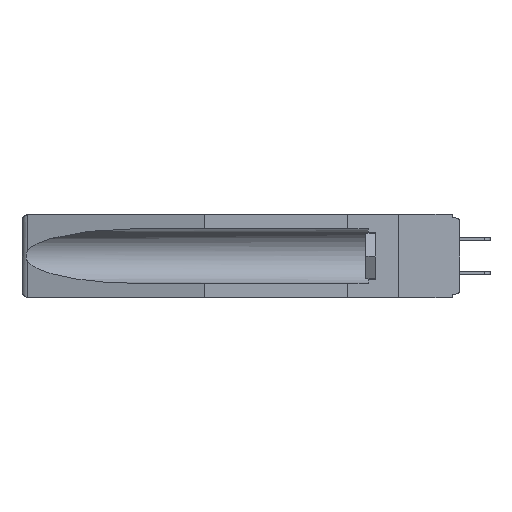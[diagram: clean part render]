
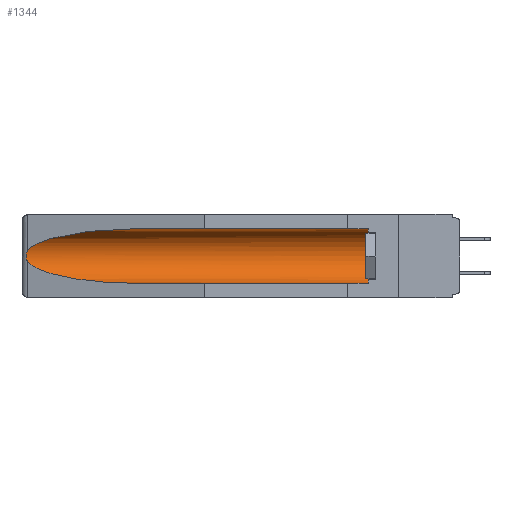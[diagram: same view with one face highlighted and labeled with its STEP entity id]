
A CAD part, left-side view. The second image highlights one B-rep face of the part: STEP entity #1344.
In plain terms, the highlighted cylindrical face has radius 2.857 mm (diameter 5.715 mm), a partial arc.
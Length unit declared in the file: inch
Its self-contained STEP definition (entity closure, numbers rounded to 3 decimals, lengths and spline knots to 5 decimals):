
#11 = LINE ( 'NONE', #16785, #6867 ) ;
#133 = CARTESIAN_POINT ( 'NONE',  ( 0.2673, 1.5327, -0.16383 ) ) ;
#203 = CARTESIAN_POINT ( 'NONE',  ( 0.2673, 1.53269, -0.17917 ) ) ;
#347 = AXIS2_PLACEMENT_3D ( 'NONE', #17643, #7484, #14903 ) ;
#1344 = ADVANCED_FACE ( 'NONE', ( #14683 ), #8242, .F. ) ;
#1616 = CARTESIAN_POINT ( 'NONE',  ( 0.2675, 1.53308, -0.17534 ) ) ;
#1624 = CARTESIAN_POINT ( 'NONE',  ( 0.26537, 1.52718, -0.19328 ) ) ;
#1692 = EDGE_CURVE ( 'NONE', #14448, #6231, #11, .T. ) ;
#2121 = CARTESIAN_POINT ( 'NONE',  ( 0.26537, 1.52718, -0.14972 ) ) ;
#2206 = CARTESIAN_POINT ( 'NONE',  ( 0.25451, 1.48313, -0.09465 ) ) ;
#2249 = DIRECTION ( 'NONE',  ( 0., 1., 0. ) ) ;
#2515 = VERTEX_POINT ( 'NONE', #17437 ) ;
#2989 = LINE ( 'NONE', #17685, #14183 ) ;
#2992 = VERTEX_POINT ( 'NONE', #1624 ) ;
#3052 = CARTESIAN_POINT ( 'NONE',  ( 0.21114, 1.30732, -0.284 ) ) ;
#4793 = CARTESIAN_POINT ( 'NONE',  ( 0.26654, 1.53092, -0.15636 ) ) ;
#5780 = CARTESIAN_POINT ( 'NONE',  ( 0.25451, 1.48313, -0.24835 ) ) ;
#6231 = VERTEX_POINT ( 'NONE', #18066 ) ;
#6867 = VECTOR ( 'NONE', #2249, 39.37008 ) ;
#6949 = VERTEX_POINT ( 'NONE', #2121 ) ;
#7407 = ORIENTED_EDGE ( 'NONE', *, *, #7430, .T. ) ;
#7430 = EDGE_CURVE ( 'NONE', #2992, #13220, #15342, .T. ) ;
#7484 = DIRECTION ( 'NONE',  ( 0., -1., 0. ) ) ;
#7545 = CARTESIAN_POINT ( 'NONE',  ( 0.26655, 1.53094, -0.18657 ) ) ;
#8242 = CYLINDRICAL_SURFACE ( 'NONE', #15646, 0.1125 ) ;
#8252 = EDGE_LOOP ( 'NONE', ( #8277, #15063, #7407, #18660, #12373, #13722 ) ) ;
#8277 = ORIENTED_EDGE ( 'NONE', *, *, #12272, .T. ) ;
#8995 = CARTESIAN_POINT ( 'NONE',  ( 0.26537, 1.52718, -0.19328 ) ) ;
#9013 = CARTESIAN_POINT ( 'NONE',  ( 0.155, 1.07973, -0.284 ) ) ;
#9361 = B_SPLINE_CURVE_WITH_KNOTS ( 'NONE', 3,
 ( #13959, #9638, #4793, #133, #10348, #1616, #203, #7545, #17821, #8995 ),
 .UNSPECIFIED., .F., .F.,
 ( 4, 2, 2, 2, 4 ),
 ( 0., 0.00029, 0.00058, 0.00087, 0.00117 ),
 .UNSPECIFIED. ) ;
#9586 = DIRECTION ( 'NONE',  ( 0., 0., 1. ) ) ;
#9638 = CARTESIAN_POINT ( 'NONE',  ( 0.26597, 1.52961, -0.15275 ) ) ;
#9913 = CARTESIAN_POINT ( 'NONE',  ( 0.155, 0.126, -0.059 ) ) ;
#10348 = CARTESIAN_POINT ( 'NONE',  ( 0.2675, 1.53308, -0.16763 ) ) ;
#10486 = EDGE_CURVE ( 'NONE', #6949, #2992, #9361, .T. ) ;
#10558 = CARTESIAN_POINT ( 'NONE',  ( 0.155, 1.07973, -0.059 ) ) ;
#11369 = EDGE_CURVE ( 'NONE', #2515, #14448, #15495, .T. ) ;
#12272 = EDGE_CURVE ( 'NONE', #6231, #6949, #12722, .T. ) ;
#12373 = ORIENTED_EDGE ( 'NONE', *, *, #11369, .T. ) ;
#12406 = CARTESIAN_POINT ( 'NONE',  ( 0.26537, 1.52718, -0.14972 ) ) ;
#12642 = EDGE_CURVE ( 'NONE', #2515, #13220, #2989, .T. ) ;
#12713 = DIRECTION ( 'NONE',  ( 0., 1., 0. ) ) ;
#12722 =( BOUNDED_CURVE ( )  B_SPLINE_CURVE ( 3, ( #10558, #16440, #2206, #12406 ),
 .UNSPECIFIED., .F., .F. ) 
 B_SPLINE_CURVE_WITH_KNOTS ( ( 4, 4 ),
 ( 4.71239, 6.08839 ),
 .UNSPECIFIED. ) 
 CURVE ( )  GEOMETRIC_REPRESENTATION_ITEM ( )  RATIONAL_B_SPLINE_CURVE ( ( 1., 0.848, 0.848, 1. ) ) 
 REPRESENTATION_ITEM ( '' )  );
#13003 = CARTESIAN_POINT ( 'NONE',  ( 0.26537, 1.52718, -0.19328 ) ) ;
#13220 = VERTEX_POINT ( 'NONE', #9013 ) ;
#13722 = ORIENTED_EDGE ( 'NONE', *, *, #1692, .T. ) ;
#13959 = CARTESIAN_POINT ( 'NONE',  ( 0.26537, 1.52718, -0.14972 ) ) ;
#14183 = VECTOR ( 'NONE', #17799, 39.37008 ) ;
#14448 = VERTEX_POINT ( 'NONE', #9913 ) ;
#14683 = FACE_OUTER_BOUND ( 'NONE', #8252, .T. ) ;
#14903 = DIRECTION ( 'NONE',  ( 0., 0., 1. ) ) ;
#15063 = ORIENTED_EDGE ( 'NONE', *, *, #10486, .T. ) ;
#15342 =( BOUNDED_CURVE ( )  B_SPLINE_CURVE ( 3, ( #13003, #5780, #3052, #17531 ),
 .UNSPECIFIED., .F., .F. ) 
 B_SPLINE_CURVE_WITH_KNOTS ( ( 4, 4 ),
 ( 0.1948, 1.5708 ),
 .UNSPECIFIED. ) 
 CURVE ( )  GEOMETRIC_REPRESENTATION_ITEM ( )  RATIONAL_B_SPLINE_CURVE ( ( 1., 0.848, 0.848, 1. ) ) 
 REPRESENTATION_ITEM ( '' )  );
#15495 = CIRCLE ( 'NONE', #347, 0.1125 ) ;
#15646 = AXIS2_PLACEMENT_3D ( 'NONE', #17185, #12713, #9586 ) ;
#16440 = CARTESIAN_POINT ( 'NONE',  ( 0.21114, 1.30732, -0.059 ) ) ;
#16785 = CARTESIAN_POINT ( 'NONE',  ( 0.155, -0.30754, -0.059 ) ) ;
#17185 = CARTESIAN_POINT ( 'NONE',  ( 0.155, -0.30754, -0.1715 ) ) ;
#17437 = CARTESIAN_POINT ( 'NONE',  ( 0.155, 0.126, -0.284 ) ) ;
#17531 = CARTESIAN_POINT ( 'NONE',  ( 0.155, 1.07973, -0.284 ) ) ;
#17643 = CARTESIAN_POINT ( 'NONE',  ( 0.155, 0.126, -0.1715 ) ) ;
#17685 = CARTESIAN_POINT ( 'NONE',  ( 0.155, -0.30754, -0.284 ) ) ;
#17799 = DIRECTION ( 'NONE',  ( 0., 1., 0. ) ) ;
#17821 = CARTESIAN_POINT ( 'NONE',  ( 0.26597, 1.5296, -0.19026 ) ) ;
#18066 = CARTESIAN_POINT ( 'NONE',  ( 0.155, 1.07973, -0.059 ) ) ;
#18660 = ORIENTED_EDGE ( 'NONE', *, *, #12642, .F. ) ;
